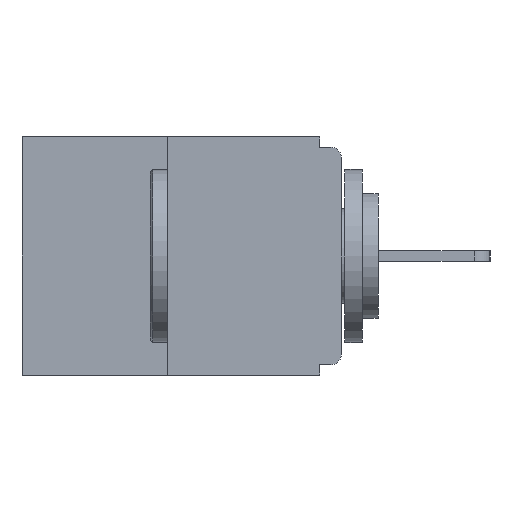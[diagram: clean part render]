
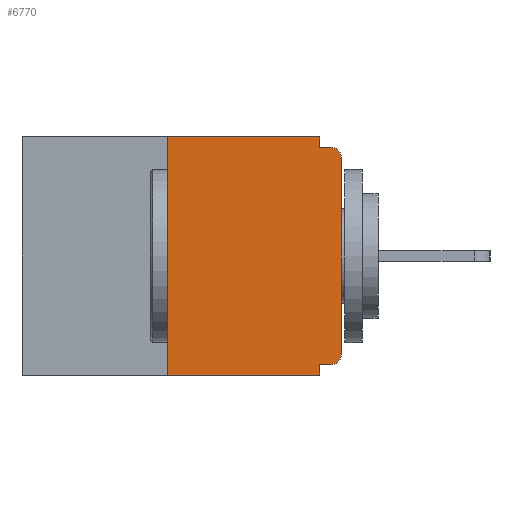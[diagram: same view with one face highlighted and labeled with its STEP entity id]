
A CAD part, left-side view. The second image highlights one B-rep face of the part: STEP entity #6770.
In plain terms, the highlighted planar face has unit normal (-1, 0, 0).
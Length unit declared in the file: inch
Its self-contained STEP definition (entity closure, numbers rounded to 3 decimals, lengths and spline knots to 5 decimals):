
#307 = VERTEX_POINT ( 'NONE', #10753 ) ;
#677 = VERTEX_POINT ( 'NONE', #1349 ) ;
#840 = DIRECTION ( 'NONE',  ( 0., 0., 1. ) ) ;
#1082 = DIRECTION ( 'NONE',  ( 0., 0., -1. ) ) ;
#1113 = CARTESIAN_POINT ( 'NONE',  ( 0., 0.031, -0.343 ) ) ;
#1349 = CARTESIAN_POINT ( 'NONE',  ( 0., 0., -0.313 ) ) ;
#1510 = EDGE_CURVE ( 'NONE', #6830, #5256, #2350, .T. ) ;
#1518 = VERTEX_POINT ( 'NONE', #12239 ) ;
#2013 = LINE ( 'NONE', #6838, #7487 ) ;
#2047 = EDGE_CURVE ( 'NONE', #1518, #307, #7451, .T. ) ;
#2284 = EDGE_CURVE ( 'NONE', #7886, #677, #4794, .T. ) ;
#2350 = CIRCLE ( 'NONE', #10430, 0.015 ) ;
#2396 = CARTESIAN_POINT ( 'NONE',  ( 0., 0.031, -0.015 ) ) ;
#2471 = VECTOR ( 'NONE', #840, 39.37008 ) ;
#2642 = FACE_OUTER_BOUND ( 'NONE', #5905, .T. ) ;
#2740 = EDGE_CURVE ( 'NONE', #10189, #307, #11177, .T. ) ;
#3077 = EDGE_CURVE ( 'NONE', #5705, #5256, #2013, .T. ) ;
#3310 = AXIS2_PLACEMENT_3D ( 'NONE', #7911, #9653, #8961 ) ;
#3416 = DIRECTION ( 'NONE',  ( 0., 1., 0. ) ) ;
#3541 = CARTESIAN_POINT ( 'NONE',  ( 0., 0., -0.328 ) ) ;
#3619 = DIRECTION ( 'NONE',  ( 0., -1., 0. ) ) ;
#3623 = AXIS2_PLACEMENT_3D ( 'NONE', #12523, #3855, #3869 ) ;
#3855 = DIRECTION ( 'NONE',  ( 1., 0., 0. ) ) ;
#3869 = DIRECTION ( 'NONE',  ( 0., 0., -1. ) ) ;
#3944 = DIRECTION ( 'NONE',  ( 0., 0., 1. ) ) ;
#4076 = CARTESIAN_POINT ( 'NONE',  ( 0., 0., 0. ) ) ;
#4135 = CARTESIAN_POINT ( 'NONE',  ( 0., 0.031, 0. ) ) ;
#4261 = CARTESIAN_POINT ( 'NONE',  ( 0., 0.25, 0. ) ) ;
#4321 = VERTEX_POINT ( 'NONE', #4135 ) ;
#4630 = VECTOR ( 'NONE', #10297, 39.37008 ) ;
#4794 = CIRCLE ( 'NONE', #3310, 0.015 ) ;
#4827 = VECTOR ( 'NONE', #3416, 39.37008 ) ;
#5256 = VERTEX_POINT ( 'NONE', #11610 ) ;
#5705 = VERTEX_POINT ( 'NONE', #2396 ) ;
#5746 = VERTEX_POINT ( 'NONE', #6535 ) ;
#5747 = VECTOR ( 'NONE', #7666, 39.37008 ) ;
#5905 = EDGE_LOOP ( 'NONE', ( #6849, #6887, #7067, #7079, #7248, #7283, #7307, #7318, #7354, #7373 ) ) ;
#6179 = LINE ( 'NONE', #4076, #11216 ) ;
#6231 = CARTESIAN_POINT ( 'NONE',  ( 0., 0.46, -0.343 ) ) ;
#6535 = CARTESIAN_POINT ( 'NONE',  ( 0., 0.25, 0. ) ) ;
#6568 = CARTESIAN_POINT ( 'NONE',  ( 0., 0.015, -0.328 ) ) ;
#6604 = CARTESIAN_POINT ( 'NONE',  ( 0., 0.031, 0. ) ) ;
#6770 = ADVANCED_FACE ( 'NONE', ( #2642 ), #12900, .F. ) ;
#6830 = VERTEX_POINT ( 'NONE', #10582 ) ;
#6838 = CARTESIAN_POINT ( 'NONE',  ( 0., 0., -0.015 ) ) ;
#6849 = ORIENTED_EDGE ( 'NONE', *, *, #7443, .F. ) ;
#6887 = ORIENTED_EDGE ( 'NONE', *, *, #11448, .F. ) ;
#7067 = ORIENTED_EDGE ( 'NONE', *, *, #2047, .T. ) ;
#7079 = ORIENTED_EDGE ( 'NONE', *, *, #2740, .F. ) ;
#7226 = VECTOR ( 'NONE', #9906, 39.37008 ) ;
#7248 = ORIENTED_EDGE ( 'NONE', *, *, #9491, .F. ) ;
#7283 = ORIENTED_EDGE ( 'NONE', *, *, #2284, .T. ) ;
#7307 = ORIENTED_EDGE ( 'NONE', *, *, #9413, .T. ) ;
#7318 = ORIENTED_EDGE ( 'NONE', *, *, #1510, .T. ) ;
#7354 = ORIENTED_EDGE ( 'NONE', *, *, #3077, .F. ) ;
#7373 = ORIENTED_EDGE ( 'NONE', *, *, #12716, .F. ) ;
#7443 = EDGE_CURVE ( 'NONE', #5746, #4321, #12200, .T. ) ;
#7451 = LINE ( 'NONE', #6231, #4630 ) ;
#7487 = VECTOR ( 'NONE', #3619, 39.37008 ) ;
#7666 = DIRECTION ( 'NONE',  ( 0., 0., -1. ) ) ;
#7886 = VERTEX_POINT ( 'NONE', #6568 ) ;
#7911 = CARTESIAN_POINT ( 'NONE',  ( 0., 0.015, -0.313 ) ) ;
#8220 = LINE ( 'NONE', #6604, #5747 ) ;
#8961 = DIRECTION ( 'NONE',  ( 0., 0., -1. ) ) ;
#9413 = EDGE_CURVE ( 'NONE', #677, #6830, #6179, .T. ) ;
#9491 = EDGE_CURVE ( 'NONE', #7886, #10189, #12931, .T. ) ;
#9653 = DIRECTION ( 'NONE',  ( -1., 0., 0. ) ) ;
#9906 = DIRECTION ( 'NONE',  ( 0., -1., 0. ) ) ;
#10189 = VERTEX_POINT ( 'NONE', #13283 ) ;
#10297 = DIRECTION ( 'NONE',  ( 0., -1., 0. ) ) ;
#10430 = AXIS2_PLACEMENT_3D ( 'NONE', #13343, #12715, #12743 ) ;
#10582 = CARTESIAN_POINT ( 'NONE',  ( 0., 0., -0.03 ) ) ;
#10753 = CARTESIAN_POINT ( 'NONE',  ( 0., 0.031, -0.343 ) ) ;
#10862 = LINE ( 'NONE', #4261, #2471 ) ;
#10881 = VECTOR ( 'NONE', #1082, 39.37008 ) ;
#11177 = LINE ( 'NONE', #1113, #10881 ) ;
#11216 = VECTOR ( 'NONE', #3944, 39.37008 ) ;
#11448 = EDGE_CURVE ( 'NONE', #1518, #5746, #10862, .T. ) ;
#11610 = CARTESIAN_POINT ( 'NONE',  ( 0., 0.015, -0.015 ) ) ;
#12200 = LINE ( 'NONE', #13248, #7226 ) ;
#12239 = CARTESIAN_POINT ( 'NONE',  ( 0., 0.25, -0.343 ) ) ;
#12523 = CARTESIAN_POINT ( 'NONE',  ( 0., 0.46, 0. ) ) ;
#12715 = DIRECTION ( 'NONE',  ( -1., 0., 0. ) ) ;
#12716 = EDGE_CURVE ( 'NONE', #4321, #5705, #8220, .T. ) ;
#12743 = DIRECTION ( 'NONE',  ( 0., 0., -1. ) ) ;
#12900 = PLANE ( 'NONE',  #3623 ) ;
#12931 = LINE ( 'NONE', #3541, #4827 ) ;
#13248 = CARTESIAN_POINT ( 'NONE',  ( 0., 0.46, 0. ) ) ;
#13283 = CARTESIAN_POINT ( 'NONE',  ( 0., 0.031, -0.328 ) ) ;
#13343 = CARTESIAN_POINT ( 'NONE',  ( 0., 0.015, -0.03 ) ) ;
